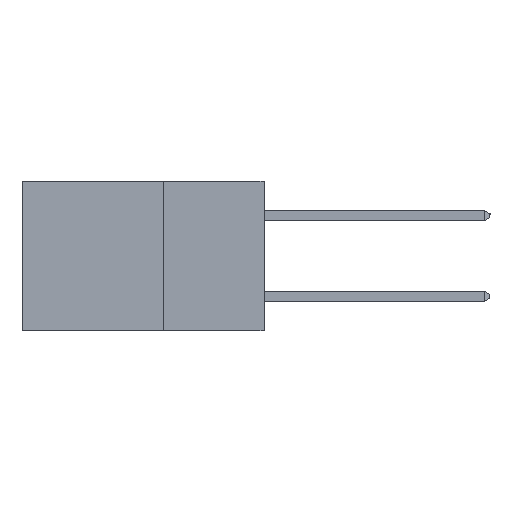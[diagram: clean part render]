
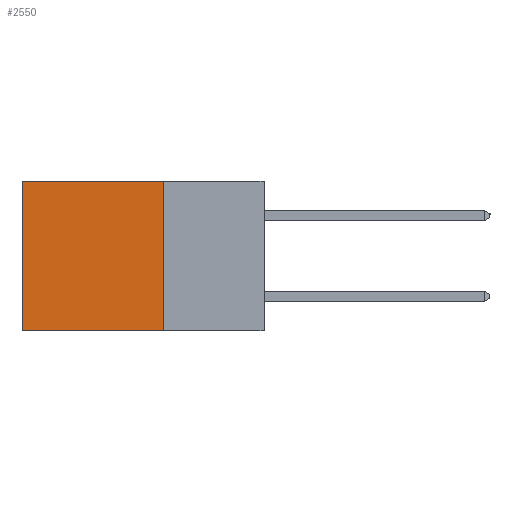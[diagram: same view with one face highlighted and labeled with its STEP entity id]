
A CAD part, left-side view. The second image highlights one B-rep face of the part: STEP entity #2550.
In plain terms, the highlighted planar face has unit normal (-1, 0, 0).
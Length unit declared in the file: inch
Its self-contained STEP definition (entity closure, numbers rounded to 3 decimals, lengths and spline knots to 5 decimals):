
#340 = DIRECTION ( 'NONE',  ( 1., 0., 0. ) ) ;
#411 = PLANE ( 'NONE',  #4383 ) ;
#551 = LINE ( 'NONE', #4849, #8727 ) ;
#770 = CARTESIAN_POINT ( 'NONE',  ( 0.2615, 0.25, 0. ) ) ;
#1329 = DIRECTION ( 'NONE',  ( 0., 0., -1. ) ) ;
#1808 = CARTESIAN_POINT ( 'NONE',  ( 0.2615, 0.6, 0. ) ) ;
#1935 = VECTOR ( 'NONE', #1329, 39.37008 ) ;
#2506 = DIRECTION ( 'NONE',  ( 0., 0., -1. ) ) ;
#2550 = ADVANCED_FACE ( 'NONE', ( #2709 ), #411, .F. ) ;
#2709 = FACE_OUTER_BOUND ( 'NONE', #12865, .T. ) ;
#3265 = VECTOR ( 'NONE', #10066, 39.37008 ) ;
#3595 = VERTEX_POINT ( 'NONE', #770 ) ;
#3743 = CARTESIAN_POINT ( 'NONE',  ( 0.2615, 0.6, -0.37 ) ) ;
#4015 = CARTESIAN_POINT ( 'NONE',  ( 0.2615, 0.25, -0.37 ) ) ;
#4090 = EDGE_CURVE ( 'NONE', #3595, #9304, #13541, .T. ) ;
#4383 = AXIS2_PLACEMENT_3D ( 'NONE', #10020, #340, #2506 ) ;
#4849 = CARTESIAN_POINT ( 'NONE',  ( 0.2615, 0.25, 0. ) ) ;
#7158 = EDGE_CURVE ( 'NONE', #9304, #12042, #11055, .T. ) ;
#7675 = LINE ( 'NONE', #10803, #1935 ) ;
#8727 = VECTOR ( 'NONE', #9053, 39.37008 ) ;
#9053 = DIRECTION ( 'NONE',  ( 0., 1., 0. ) ) ;
#9233 = ORIENTED_EDGE ( 'NONE', *, *, #11886, .T. ) ;
#9304 = VERTEX_POINT ( 'NONE', #13127 ) ;
#10020 = CARTESIAN_POINT ( 'NONE',  ( 0.2615, 0.25, -0.37 ) ) ;
#10066 = DIRECTION ( 'NONE',  ( 0., 1., 0. ) ) ;
#10150 = ORIENTED_EDGE ( 'NONE', *, *, #4090, .F. ) ;
#10725 = VECTOR ( 'NONE', #11419, 39.37008 ) ;
#10803 = CARTESIAN_POINT ( 'NONE',  ( 0.2615, 0.6, -0.37 ) ) ;
#11055 = LINE ( 'NONE', #12248, #3265 ) ;
#11184 = ORIENTED_EDGE ( 'NONE', *, *, #7158, .F. ) ;
#11419 = DIRECTION ( 'NONE',  ( 0., 0., -1. ) ) ;
#11544 = ORIENTED_EDGE ( 'NONE', *, *, #12035, .T. ) ;
#11886 = EDGE_CURVE ( 'NONE', #12098, #12042, #7675, .T. ) ;
#12035 = EDGE_CURVE ( 'NONE', #3595, #12098, #551, .T. ) ;
#12042 = VERTEX_POINT ( 'NONE', #3743 ) ;
#12098 = VERTEX_POINT ( 'NONE', #1808 ) ;
#12248 = CARTESIAN_POINT ( 'NONE',  ( 0.2615, 0.25, -0.37 ) ) ;
#12865 = EDGE_LOOP ( 'NONE', ( #9233, #11184, #10150, #11544 ) ) ;
#13127 = CARTESIAN_POINT ( 'NONE',  ( 0.2615, 0.25, -0.37 ) ) ;
#13541 = LINE ( 'NONE', #4015, #10725 ) ;
